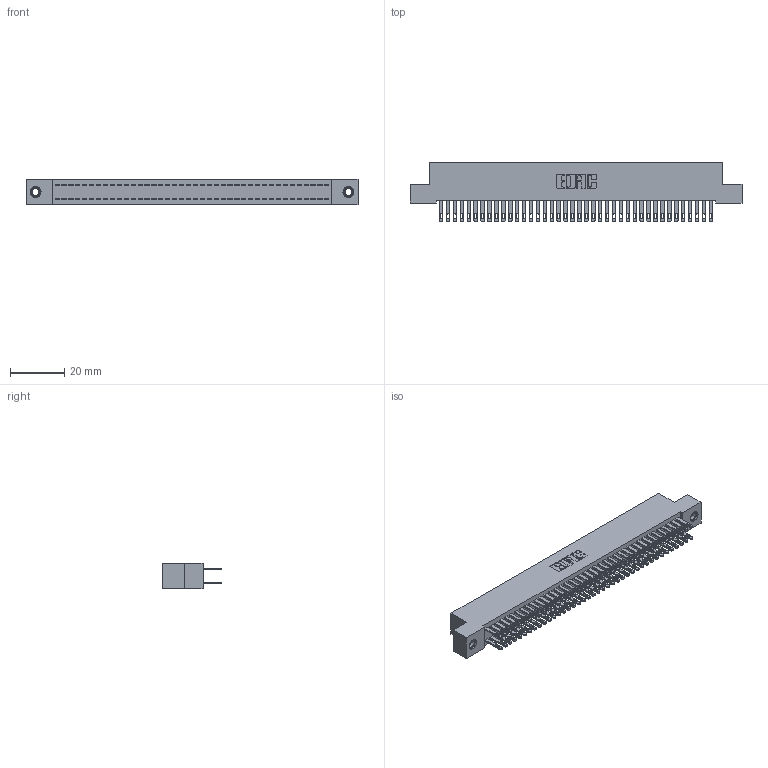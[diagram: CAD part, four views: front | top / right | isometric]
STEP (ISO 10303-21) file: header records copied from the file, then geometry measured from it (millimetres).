
FILE_DESCRIPTION (( 'STEP AP203' ), '1' );
FILE_NAME ('342-080-500-207.STEP', '2019-10-04T11:28:32', ( '' ), ( '' ), 'SwSTEP 2.0', 'SolidWorks 2016', '' );
FILE_SCHEMA (( 'CONFIG_CONTROL_DESIGN' ));
Length unit declared in the file: inch
Products named in the file (4): 342 Part_TI; 345-292-001_345-293-100; 345-250-001_345-250-005-103; 342-080-500-207
Assembly tree (83 placements, depth 2):
  342-080-500-207
    342 Part_TI
    345-292-001_345-293-100  x80
    345-250-001_345-250-005-103  x2
Bounding box: 121.92 x 21.85 x 9.4 mm (x, y, z)
Volume: 11176.8 mm3; surface area: 18935.5 mm2
Topology: 83 solids, 83 shells, 4010 faces, 12195 edges, 8122 vertices
Faces by surface type: plane 2498, cylinder 1496, cone 12, torus 4
Entity records: 26976 total; most frequent: CARTESIAN_POINT 4453, ORIENTED_EDGE 4382, DIRECTION 3841, EDGE_CURVE 2191, LINE 2039, VECTOR 2039, VERTEX_POINT 1456, AXIS2_PLACEMENT_3D 901
